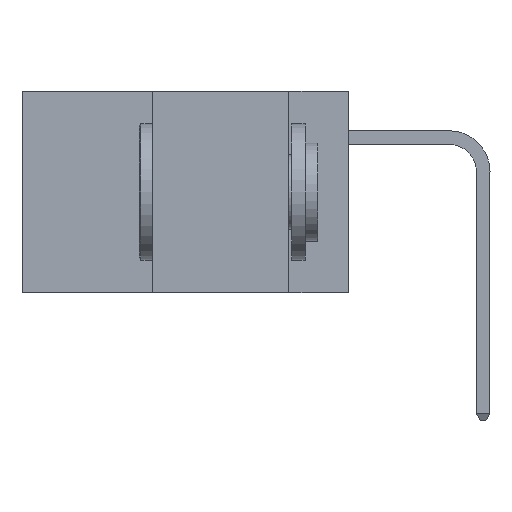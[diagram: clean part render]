
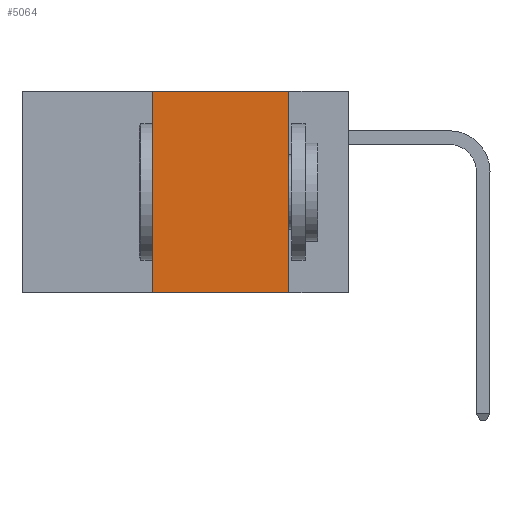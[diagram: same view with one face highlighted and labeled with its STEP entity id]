
A CAD part, left-side view. The second image highlights one B-rep face of the part: STEP entity #5064.
In plain terms, the highlighted planar face has unit normal (-1, 0, 0).
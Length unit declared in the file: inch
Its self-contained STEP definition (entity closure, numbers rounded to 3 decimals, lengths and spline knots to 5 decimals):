
#565 = EDGE_CURVE ( 'NONE', #3264, #7923, #2630, .T. ) ;
#620 = VERTEX_POINT ( 'NONE', #8160 ) ;
#777 = EDGE_CURVE ( 'NONE', #620, #3264, #1007, .T. ) ;
#858 = DIRECTION ( 'NONE',  ( 0., -1., 0. ) ) ;
#1007 = LINE ( 'NONE', #1714, #1560 ) ;
#1341 = VERTEX_POINT ( 'NONE', #4134 ) ;
#1519 = EDGE_LOOP ( 'NONE', ( #3158, #5667, #4088, #9059 ) ) ;
#1560 = VECTOR ( 'NONE', #2760, 39.37008 ) ;
#1600 = PLANE ( 'NONE',  #6317 ) ;
#1714 = CARTESIAN_POINT ( 'NONE',  ( 0., 0.36, 0. ) ) ;
#2435 = VECTOR ( 'NONE', #6275, 39.37008 ) ;
#2630 = LINE ( 'NONE', #10241, #2435 ) ;
#2675 = DIRECTION ( 'NONE',  ( 0., 0., -1. ) ) ;
#2760 = DIRECTION ( 'NONE',  ( 0., 0., 1. ) ) ;
#2935 = CARTESIAN_POINT ( 'NONE',  ( 0., 0.11, 0. ) ) ;
#3087 = FACE_OUTER_BOUND ( 'NONE', #1519, .T. ) ;
#3158 = ORIENTED_EDGE ( 'NONE', *, *, #7944, .F. ) ;
#3264 = VERTEX_POINT ( 'NONE', #3740 ) ;
#3740 = CARTESIAN_POINT ( 'NONE',  ( 0., 0.36, 0. ) ) ;
#4088 = ORIENTED_EDGE ( 'NONE', *, *, #777, .F. ) ;
#4134 = CARTESIAN_POINT ( 'NONE',  ( 0., 0.11, -0.37 ) ) ;
#4700 = EDGE_CURVE ( 'NONE', #620, #1341, #8563, .T. ) ;
#5064 = ADVANCED_FACE ( 'NONE', ( #3087 ), #1600, .F. ) ;
#5667 = ORIENTED_EDGE ( 'NONE', *, *, #565, .F. ) ;
#6275 = DIRECTION ( 'NONE',  ( 0., -1., 0. ) ) ;
#6317 = AXIS2_PLACEMENT_3D ( 'NONE', #6332, #7918, #2675 ) ;
#6332 = CARTESIAN_POINT ( 'NONE',  ( 0., 0.6, 0. ) ) ;
#7040 = VECTOR ( 'NONE', #9570, 39.37008 ) ;
#7239 = LINE ( 'NONE', #2935, #7040 ) ;
#7918 = DIRECTION ( 'NONE',  ( 1., 0., 0. ) ) ;
#7923 = VERTEX_POINT ( 'NONE', #8745 ) ;
#7944 = EDGE_CURVE ( 'NONE', #7923, #1341, #7239, .T. ) ;
#8079 = CARTESIAN_POINT ( 'NONE',  ( 0., 0.6, -0.37 ) ) ;
#8160 = CARTESIAN_POINT ( 'NONE',  ( 0., 0.36, -0.37 ) ) ;
#8562 = VECTOR ( 'NONE', #858, 39.37008 ) ;
#8563 = LINE ( 'NONE', #8079, #8562 ) ;
#8745 = CARTESIAN_POINT ( 'NONE',  ( 0., 0.11, 0. ) ) ;
#9059 = ORIENTED_EDGE ( 'NONE', *, *, #4700, .T. ) ;
#9570 = DIRECTION ( 'NONE',  ( 0., 0., -1. ) ) ;
#10241 = CARTESIAN_POINT ( 'NONE',  ( 0., 0.6, 0. ) ) ;
